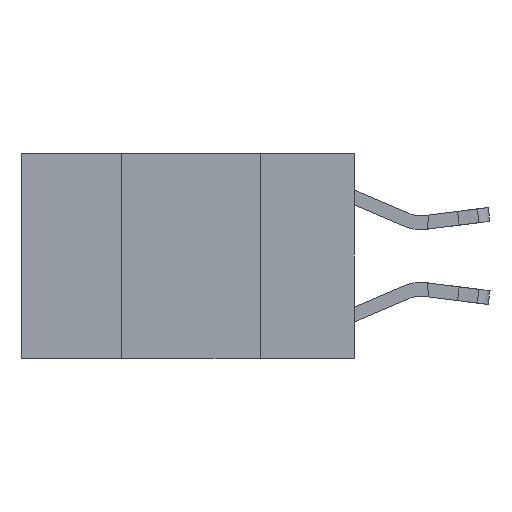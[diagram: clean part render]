
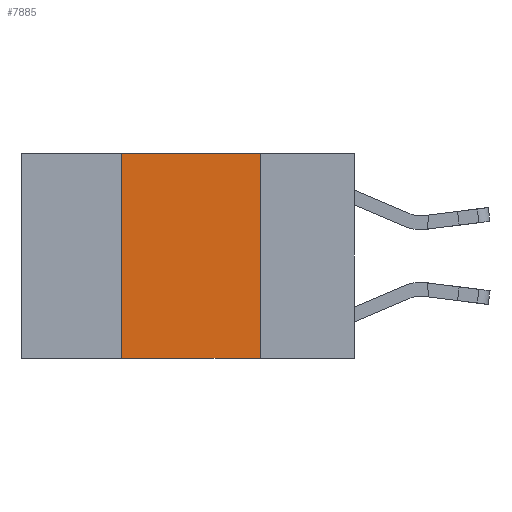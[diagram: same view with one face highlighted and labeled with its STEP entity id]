
A CAD part, left-side view. The second image highlights one B-rep face of the part: STEP entity #7885.
In plain terms, the highlighted planar face has unit normal (-1, 0, 0).
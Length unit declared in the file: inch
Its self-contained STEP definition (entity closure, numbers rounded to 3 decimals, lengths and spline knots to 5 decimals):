
#15 = VERTEX_POINT ( 'NONE', #1988 ) ;
#53 = CARTESIAN_POINT ( 'NONE',  ( 0., 0.42, 0. ) ) ;
#195 = VERTEX_POINT ( 'NONE', #53 ) ;
#655 = ORIENTED_EDGE ( 'NONE', *, *, #6748, .F. ) ;
#813 = VECTOR ( 'NONE', #1253, 39.37008 ) ;
#1077 = DIRECTION ( 'NONE',  ( 0., 0., 1. ) ) ;
#1156 = LINE ( 'NONE', #6552, #813 ) ;
#1253 = DIRECTION ( 'NONE',  ( 0., -1., 0. ) ) ;
#1409 = EDGE_CURVE ( 'NONE', #15, #2618, #7006, .T. ) ;
#1988 = CARTESIAN_POINT ( 'NONE',  ( 0., 0.42, -0.37 ) ) ;
#2618 = VERTEX_POINT ( 'NONE', #7107 ) ;
#2861 = DIRECTION ( 'NONE',  ( 0., 0., -1. ) ) ;
#3223 = FACE_OUTER_BOUND ( 'NONE', #3255, .T. ) ;
#3255 = EDGE_LOOP ( 'NONE', ( #4070, #3686, #655, #13163 ) ) ;
#3686 = ORIENTED_EDGE ( 'NONE', *, *, #13823, .F. ) ;
#3858 = VECTOR ( 'NONE', #6140, 39.37008 ) ;
#4070 = ORIENTED_EDGE ( 'NONE', *, *, #13139, .F. ) ;
#4089 = VECTOR ( 'NONE', #1077, 39.37008 ) ;
#4138 = PLANE ( 'NONE',  #4569 ) ;
#4569 = AXIS2_PLACEMENT_3D ( 'NONE', #11743, #5216, #12864 ) ;
#5216 = DIRECTION ( 'NONE',  ( 1., 0., 0. ) ) ;
#6140 = DIRECTION ( 'NONE',  ( 0., -1., 0. ) ) ;
#6552 = CARTESIAN_POINT ( 'NONE',  ( 0., 0.6, 0. ) ) ;
#6748 = EDGE_CURVE ( 'NONE', #15, #195, #6910, .T. ) ;
#6910 = LINE ( 'NONE', #8594, #4089 ) ;
#7006 = LINE ( 'NONE', #13831, #3858 ) ;
#7107 = CARTESIAN_POINT ( 'NONE',  ( 0., 0.17, -0.37 ) ) ;
#7174 = LINE ( 'NONE', #8210, #9837 ) ;
#7885 = ADVANCED_FACE ( 'NONE', ( #3223 ), #4138, .F. ) ;
#8210 = CARTESIAN_POINT ( 'NONE',  ( 0., 0.17, 0. ) ) ;
#8594 = CARTESIAN_POINT ( 'NONE',  ( 0., 0.42, 0. ) ) ;
#9837 = VECTOR ( 'NONE', #2861, 39.37008 ) ;
#10720 = CARTESIAN_POINT ( 'NONE',  ( 0., 0.17, 0. ) ) ;
#11743 = CARTESIAN_POINT ( 'NONE',  ( 0., 0.6, 0. ) ) ;
#12715 = VERTEX_POINT ( 'NONE', #10720 ) ;
#12864 = DIRECTION ( 'NONE',  ( 0., 0., -1. ) ) ;
#13139 = EDGE_CURVE ( 'NONE', #12715, #2618, #7174, .T. ) ;
#13163 = ORIENTED_EDGE ( 'NONE', *, *, #1409, .T. ) ;
#13823 = EDGE_CURVE ( 'NONE', #195, #12715, #1156, .T. ) ;
#13831 = CARTESIAN_POINT ( 'NONE',  ( 0., 0.6, -0.37 ) ) ;
